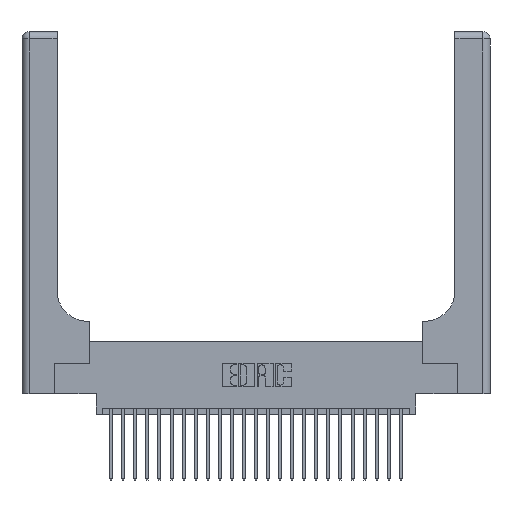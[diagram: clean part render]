
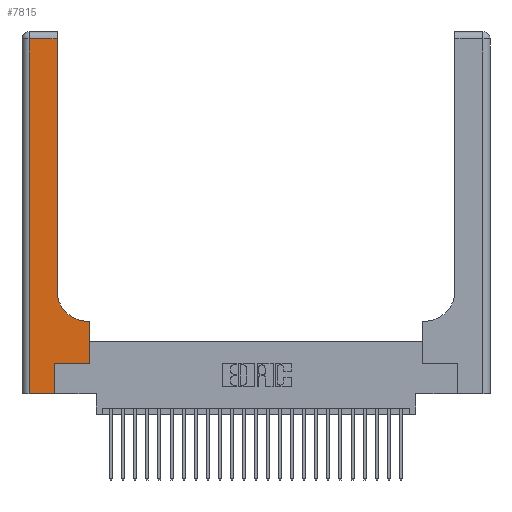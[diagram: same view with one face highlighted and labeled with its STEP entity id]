
A CAD part, top view. The second image highlights one B-rep face of the part: STEP entity #7815.
In plain terms, the highlighted planar face has unit normal (0, 0, 1).
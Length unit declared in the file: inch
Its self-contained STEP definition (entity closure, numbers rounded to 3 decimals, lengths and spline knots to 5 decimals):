
#128 = ORIENTED_EDGE ( 'NONE', *, *, #6895, .T. ) ;
#395 = VECTOR ( 'NONE', #4480, 39.37008 ) ;
#461 = CARTESIAN_POINT ( 'NONE',  ( 0.2915, 0.6, 0.37 ) ) ;
#682 = CARTESIAN_POINT ( 'NONE',  ( 0.269, 0.25, 0.37 ) ) ;
#699 = CARTESIAN_POINT ( 'NONE',  ( 0.5415, 0.6, 0.37 ) ) ;
#886 = CARTESIAN_POINT ( 'NONE',  ( 0.2915, 3., 0.37 ) ) ;
#1149 = LINE ( 'NONE', #3513, #13359 ) ;
#2268 = EDGE_LOOP ( 'NONE', ( #20719, #17015, #18986, #16420, #7390, #128, #10414, #16857, #24942 ) ) ;
#2292 = FACE_OUTER_BOUND ( 'NONE', #2268, .T. ) ;
#2415 = VECTOR ( 'NONE', #11823, 39.37008 ) ;
#2418 = DIRECTION ( 'NONE',  ( 0., 0., -1. ) ) ;
#2436 = CARTESIAN_POINT ( 'NONE',  ( 0.06, 3., 0.37 ) ) ;
#2505 = DIRECTION ( 'NONE',  ( 0., 1., 0. ) ) ;
#3513 = CARTESIAN_POINT ( 'NONE',  ( 0., 0., 0.37 ) ) ;
#4003 = LINE ( 'NONE', #12851, #395 ) ;
#4480 = DIRECTION ( 'NONE',  ( 1., 0., 0. ) ) ;
#4531 = CARTESIAN_POINT ( 'NONE',  ( 0.269, 0., 0.37 ) ) ;
#4624 = CARTESIAN_POINT ( 'NONE',  ( 0.5415, 0.85, 0.37 ) ) ;
#4633 = VECTOR ( 'NONE', #8176, 39.37008 ) ;
#5930 = EDGE_CURVE ( 'NONE', #20219, #26551, #8050, .T. ) ;
#6058 = VERTEX_POINT ( 'NONE', #14936 ) ;
#6094 = VECTOR ( 'NONE', #2505, 39.37008 ) ;
#6302 = VERTEX_POINT ( 'NONE', #15397 ) ;
#6895 = EDGE_CURVE ( 'NONE', #19670, #15733, #4003, .T. ) ;
#7390 = ORIENTED_EDGE ( 'NONE', *, *, #13721, .T. ) ;
#7406 = LINE ( 'NONE', #4531, #8752 ) ;
#7500 = AXIS2_PLACEMENT_3D ( 'NONE', #18157, #20459, #13949 ) ;
#7737 = LINE ( 'NONE', #14925, #6094 ) ;
#7815 = ADVANCED_FACE ( 'NONE', ( #2292 ), #16124, .F. ) ;
#8050 = LINE ( 'NONE', #461, #2415 ) ;
#8176 = DIRECTION ( 'NONE',  ( 0., -1., 0. ) ) ;
#8192 = LINE ( 'NONE', #8607, #19647 ) ;
#8607 = CARTESIAN_POINT ( 'NONE',  ( 0., 2.94, 0.37 ) ) ;
#8752 = VECTOR ( 'NONE', #17120, 39.37008 ) ;
#8908 = VERTEX_POINT ( 'NONE', #12274 ) ;
#9233 = VERTEX_POINT ( 'NONE', #17801 ) ;
#9363 = DIRECTION ( 'NONE',  ( 0., 1., 0. ) ) ;
#10414 = ORIENTED_EDGE ( 'NONE', *, *, #13662, .T. ) ;
#11823 = DIRECTION ( 'NONE',  ( -1., 0., 0. ) ) ;
#12274 = CARTESIAN_POINT ( 'NONE',  ( 0.2915, 0.85, 0.37 ) ) ;
#12713 = CIRCLE ( 'NONE', #22612, 0.25 ) ;
#12851 = CARTESIAN_POINT ( 'NONE',  ( 0.269, 0.25, 0.37 ) ) ;
#12940 = VERTEX_POINT ( 'NONE', #25922 ) ;
#13142 = EDGE_CURVE ( 'NONE', #8908, #12940, #15971, .T. ) ;
#13359 = VECTOR ( 'NONE', #18316, 39.37008 ) ;
#13662 = EDGE_CURVE ( 'NONE', #15733, #20219, #7737, .T. ) ;
#13721 = EDGE_CURVE ( 'NONE', #6302, #19670, #7406, .T. ) ;
#13949 = DIRECTION ( 'NONE',  ( -1., 0., 0. ) ) ;
#14645 = CARTESIAN_POINT ( 'NONE',  ( 0.5585, 0.6, 0.37 ) ) ;
#14925 = CARTESIAN_POINT ( 'NONE',  ( 0.5585, 0.25, 0.37 ) ) ;
#14936 = CARTESIAN_POINT ( 'NONE',  ( 0.06, 0., 0.37 ) ) ;
#15397 = CARTESIAN_POINT ( 'NONE',  ( 0.269, 0., 0.37 ) ) ;
#15733 = VERTEX_POINT ( 'NONE', #19206 ) ;
#15971 = LINE ( 'NONE', #886, #19576 ) ;
#16124 = PLANE ( 'NONE',  #7500 ) ;
#16420 = ORIENTED_EDGE ( 'NONE', *, *, #19778, .T. ) ;
#16857 = ORIENTED_EDGE ( 'NONE', *, *, #5930, .T. ) ;
#16904 = EDGE_CURVE ( 'NONE', #9233, #6058, #21394, .T. ) ;
#17015 = ORIENTED_EDGE ( 'NONE', *, *, #24885, .T. ) ;
#17120 = DIRECTION ( 'NONE',  ( 0., 1., 0. ) ) ;
#17801 = CARTESIAN_POINT ( 'NONE',  ( 0.06, 2.94, 0.37 ) ) ;
#18157 = CARTESIAN_POINT ( 'NONE',  ( 0., 3., 0.37 ) ) ;
#18316 = DIRECTION ( 'NONE',  ( 1., 0., 0. ) ) ;
#18986 = ORIENTED_EDGE ( 'NONE', *, *, #16904, .T. ) ;
#19206 = CARTESIAN_POINT ( 'NONE',  ( 0.5585, 0.25, 0.37 ) ) ;
#19576 = VECTOR ( 'NONE', #9363, 39.37008 ) ;
#19647 = VECTOR ( 'NONE', #23305, 39.37008 ) ;
#19670 = VERTEX_POINT ( 'NONE', #682 ) ;
#19778 = EDGE_CURVE ( 'NONE', #6058, #6302, #1149, .T. ) ;
#20219 = VERTEX_POINT ( 'NONE', #14645 ) ;
#20459 = DIRECTION ( 'NONE',  ( 0., 0., -1. ) ) ;
#20719 = ORIENTED_EDGE ( 'NONE', *, *, #13142, .T. ) ;
#21394 = LINE ( 'NONE', #2436, #4633 ) ;
#22612 = AXIS2_PLACEMENT_3D ( 'NONE', #4624, #2418, #24230 ) ;
#23305 = DIRECTION ( 'NONE',  ( -1., 0., 0. ) ) ;
#24230 = DIRECTION ( 'NONE',  ( 1., 0., 0. ) ) ;
#24885 = EDGE_CURVE ( 'NONE', #12940, #9233, #8192, .T. ) ;
#24942 = ORIENTED_EDGE ( 'NONE', *, *, #27039, .T. ) ;
#25922 = CARTESIAN_POINT ( 'NONE',  ( 0.2915, 2.94, 0.37 ) ) ;
#26551 = VERTEX_POINT ( 'NONE', #699 ) ;
#27039 = EDGE_CURVE ( 'NONE', #26551, #8908, #12713, .T. ) ;
